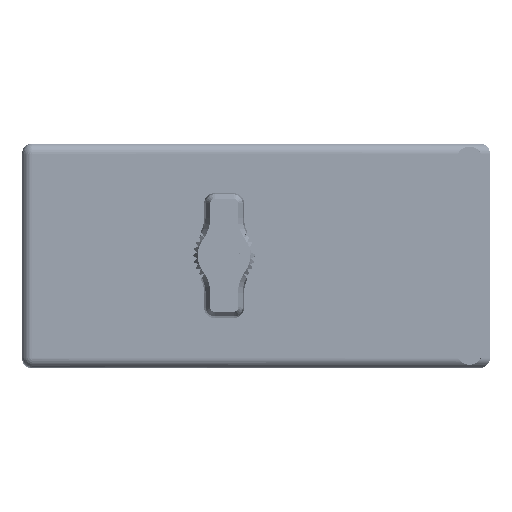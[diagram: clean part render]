
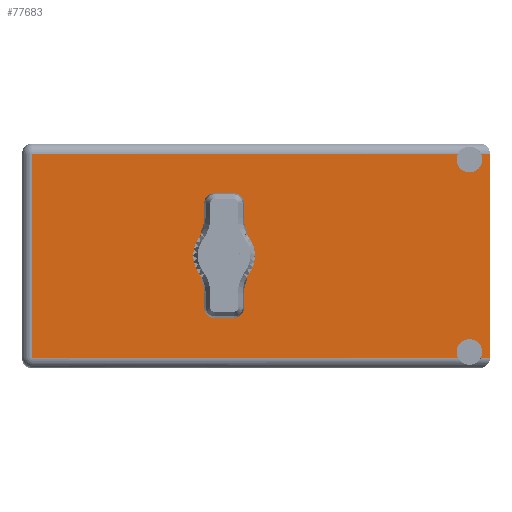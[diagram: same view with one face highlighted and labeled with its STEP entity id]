
A CAD part, top view. The second image highlights one B-rep face of the part: STEP entity #77683.
In plain terms, the highlighted face is planar.
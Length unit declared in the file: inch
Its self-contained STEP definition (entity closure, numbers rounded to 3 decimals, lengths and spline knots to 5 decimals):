
#469 = EDGE_CURVE ( 'NONE', #72061, #72449, #75913, .T. ) ;
#696 = AXIS2_PLACEMENT_3D ( 'NONE', #63739, #64887, #18447 ) ;
#1839 = EDGE_CURVE ( 'NONE', #19205, #53230, #54288, .T. ) ;
#4507 = AXIS2_PLACEMENT_3D ( 'NONE', #98380, #107230, #72317 ) ;
#10084 = EDGE_CURVE ( 'NONE', #112399, #41636, #88321, .T. ) ;
#14199 = DIRECTION ( 'NONE',  ( 0., 1., 0. ) ) ;
#14671 = CARTESIAN_POINT ( 'NONE',  ( 1.3775, 2.03, -0.595 ) ) ;
#15173 = CARTESIAN_POINT ( 'NONE',  ( 1.3775, 2.03, -0.765 ) ) ;
#15461 = CARTESIAN_POINT ( 'NONE',  ( 3.05, 2.03, -0.109 ) ) ;
#16073 = VECTOR ( 'NONE', #44898, 39.37008 ) ;
#16359 = DIRECTION ( 'NONE',  ( 0., 1., 0. ) ) ;
#16806 = EDGE_CURVE ( 'NONE', #106029, #72449, #50184, .T. ) ;
#18048 = DIRECTION ( 'NONE',  ( 1., 0., 0. ) ) ;
#18447 = DIRECTION ( 'NONE',  ( 0., 0., 1. ) ) ;
#19205 = VERTEX_POINT ( 'NONE', #24782 ) ;
#22062 = CARTESIAN_POINT ( 'NONE',  ( 3.12833, 2.03, -1.46 ) ) ;
#23466 = DIRECTION ( 'NONE',  ( 0., 0., 1. ) ) ;
#23951 = ORIENTED_EDGE ( 'NONE', *, *, #469, .F. ) ;
#24782 = CARTESIAN_POINT ( 'NONE',  ( 1.3775, 2.03, -0.935 ) ) ;
#25240 = AXIS2_PLACEMENT_3D ( 'NONE', #72967, #35763, #62974 ) ;
#25827 = VERTEX_POINT ( 'NONE', #104679 ) ;
#27542 = VECTOR ( 'NONE', #66416, 39.37008 ) ;
#29741 = CARTESIAN_POINT ( 'NONE',  ( 3.19, 2.03, 0. ) ) ;
#30900 = VECTOR ( 'NONE', #65478, 39.37008 ) ;
#33658 = DIRECTION ( 'NONE',  ( 0., 0., 1. ) ) ;
#34957 = CARTESIAN_POINT ( 'NONE',  ( 0., 2.03, -1.46 ) ) ;
#35763 = DIRECTION ( 'NONE',  ( 0., 1., 0. ) ) ;
#38375 = CARTESIAN_POINT ( 'NONE',  ( 3.05, 2.03, -0.1965 ) ) ;
#40526 = EDGE_CURVE ( 'NONE', #109167, #112399, #113701, .T. ) ;
#41636 = VERTEX_POINT ( 'NONE', #86797 ) ;
#41774 = EDGE_CURVE ( 'NONE', #109167, #64783, #76337, .T. ) ;
#44898 = DIRECTION ( 'NONE',  ( -1., 0., 0. ) ) ;
#46947 = CIRCLE ( 'NONE', #84502, 0.17 ) ;
#47622 = CARTESIAN_POINT ( 'NONE',  ( 3.12833, 2.03, -0.07 ) ) ;
#47646 = EDGE_CURVE ( 'NONE', #41636, #25827, #55198, .T. ) ;
#49614 = ORIENTED_EDGE ( 'NONE', *, *, #82512, .F. ) ;
#50184 = LINE ( 'NONE', #64106, #96099 ) ;
#53034 = ORIENTED_EDGE ( 'NONE', *, *, #96127, .F. ) ;
#53049 = ORIENTED_EDGE ( 'NONE', *, *, #10084, .T. ) ;
#53230 = VERTEX_POINT ( 'NONE', #14671 ) ;
#53412 = AXIS2_PLACEMENT_3D ( 'NONE', #111921, #93032, #93420 ) ;
#54288 = CIRCLE ( 'NONE', #66010, 0.17 ) ;
#54544 = EDGE_CURVE ( 'NONE', #72061, #115784, #103623, .T. ) ;
#55198 = LINE ( 'NONE', #74692, #30900 ) ;
#56366 = FACE_BOUND ( 'NONE', #89541, .T. ) ;
#56707 = ORIENTED_EDGE ( 'NONE', *, *, #54544, .T. ) ;
#57160 = ORIENTED_EDGE ( 'NONE', *, *, #1839, .F. ) ;
#58119 = CIRCLE ( 'NONE', #25240, 0.0875 ) ;
#62838 = CARTESIAN_POINT ( 'NONE',  ( 3.19, 2.03, -0.07 ) ) ;
#62974 = DIRECTION ( 'NONE',  ( 0., 0., 1. ) ) ;
#63739 = CARTESIAN_POINT ( 'NONE',  ( 3.05, 2.03, -1.421 ) ) ;
#64106 = CARTESIAN_POINT ( 'NONE',  ( 3.19, 2.03, -0.07 ) ) ;
#64783 = VERTEX_POINT ( 'NONE', #74119 ) ;
#64887 = DIRECTION ( 'NONE',  ( 0., 1., 0. ) ) ;
#65313 = ORIENTED_EDGE ( 'NONE', *, *, #47646, .T. ) ;
#65478 = DIRECTION ( 'NONE',  ( 1., 0., 0. ) ) ;
#65745 = DIRECTION ( 'NONE',  ( 0., 0., 1. ) ) ;
#66010 = AXIS2_PLACEMENT_3D ( 'NONE', #79571, #14199, #23466 ) ;
#66207 = CARTESIAN_POINT ( 'NONE',  ( 2.97167, 2.03, -1.46 ) ) ;
#66416 = DIRECTION ( 'NONE',  ( -1., 0., 0. ) ) ;
#68897 = ORIENTED_EDGE ( 'NONE', *, *, #16806, .T. ) ;
#72061 = VERTEX_POINT ( 'NONE', #85743 ) ;
#72317 = DIRECTION ( 'NONE',  ( 0., 0., 1. ) ) ;
#72449 = VERTEX_POINT ( 'NONE', #62838 ) ;
#72967 = CARTESIAN_POINT ( 'NONE',  ( 3.05, 2.03, -0.109 ) ) ;
#73097 = ORIENTED_EDGE ( 'NONE', *, *, #116754, .F. ) ;
#74119 = CARTESIAN_POINT ( 'NONE',  ( 3.05, 2.03, -1.3335 ) ) ;
#74692 = CARTESIAN_POINT ( 'NONE',  ( 3.19, 2.03, -0.07 ) ) ;
#75913 = LINE ( 'NONE', #29741, #101759 ) ;
#76337 = CIRCLE ( 'NONE', #4507, 0.0875 ) ;
#76574 = CIRCLE ( 'NONE', #696, 0.0875 ) ;
#77683 = ADVANCED_FACE ( 'NONE', ( #56366, #117950 ), #83442, .T. ) ;
#78827 = DIRECTION ( 'NONE',  ( 0., 1., 0. ) ) ;
#79571 = CARTESIAN_POINT ( 'NONE',  ( 1.3775, 2.03, -0.765 ) ) ;
#82512 = EDGE_CURVE ( 'NONE', #64783, #115784, #76574, .T. ) ;
#83442 = PLANE ( 'NONE',  #53412 ) ;
#84502 = AXIS2_PLACEMENT_3D ( 'NONE', #15173, #16359, #33658 ) ;
#85743 = CARTESIAN_POINT ( 'NONE',  ( 3.19, 2.03, -1.46 ) ) ;
#86556 = VERTEX_POINT ( 'NONE', #38375 ) ;
#86797 = CARTESIAN_POINT ( 'NONE',  ( 0.07, 2.03, -0.07 ) ) ;
#87219 = CARTESIAN_POINT ( 'NONE',  ( 0.07, 2.03, -1.53 ) ) ;
#88321 = LINE ( 'NONE', #87219, #89796 ) ;
#88412 = DIRECTION ( 'NONE',  ( 0., 0., 1. ) ) ;
#89541 = EDGE_LOOP ( 'NONE', ( #95218, #57160 ) ) ;
#89796 = VECTOR ( 'NONE', #88412, 39.37008 ) ;
#93032 = DIRECTION ( 'NONE',  ( 0., 1., 0. ) ) ;
#93420 = DIRECTION ( 'NONE',  ( 0., 0., 1. ) ) ;
#94190 = EDGE_CURVE ( 'NONE', #53230, #19205, #46947, .T. ) ;
#95218 = ORIENTED_EDGE ( 'NONE', *, *, #94190, .F. ) ;
#96099 = VECTOR ( 'NONE', #18048, 39.37008 ) ;
#96127 = EDGE_CURVE ( 'NONE', #86556, #25827, #106856, .T. ) ;
#97297 = ORIENTED_EDGE ( 'NONE', *, *, #40526, .T. ) ;
#98380 = CARTESIAN_POINT ( 'NONE',  ( 3.05, 2.03, -1.421 ) ) ;
#101759 = VECTOR ( 'NONE', #65745, 39.37008 ) ;
#103623 = LINE ( 'NONE', #111378, #27542 ) ;
#104679 = CARTESIAN_POINT ( 'NONE',  ( 2.97167, 2.03, -0.07 ) ) ;
#105837 = ORIENTED_EDGE ( 'NONE', *, *, #41774, .F. ) ;
#106029 = VERTEX_POINT ( 'NONE', #47622 ) ;
#106856 = CIRCLE ( 'NONE', #110030, 0.0875 ) ;
#106865 = EDGE_LOOP ( 'NONE', ( #65313, #53034, #73097, #68897, #23951, #56707, #49614, #105837, #97297, #53049 ) ) ;
#107230 = DIRECTION ( 'NONE',  ( 0., 1., 0. ) ) ;
#107686 = DIRECTION ( 'NONE',  ( 0., 0., 1. ) ) ;
#109167 = VERTEX_POINT ( 'NONE', #66207 ) ;
#110030 = AXIS2_PLACEMENT_3D ( 'NONE', #15461, #78827, #107686 ) ;
#110645 = CARTESIAN_POINT ( 'NONE',  ( 0.07, 2.03, -1.46 ) ) ;
#111378 = CARTESIAN_POINT ( 'NONE',  ( 0., 2.03, -1.46 ) ) ;
#111921 = CARTESIAN_POINT ( 'NONE',  ( 0., 2.03, -1.53 ) ) ;
#112399 = VERTEX_POINT ( 'NONE', #110645 ) ;
#113701 = LINE ( 'NONE', #34957, #16073 ) ;
#115784 = VERTEX_POINT ( 'NONE', #22062 ) ;
#116754 = EDGE_CURVE ( 'NONE', #106029, #86556, #58119, .T. ) ;
#117950 = FACE_OUTER_BOUND ( 'NONE', #106865, .T. ) ;
